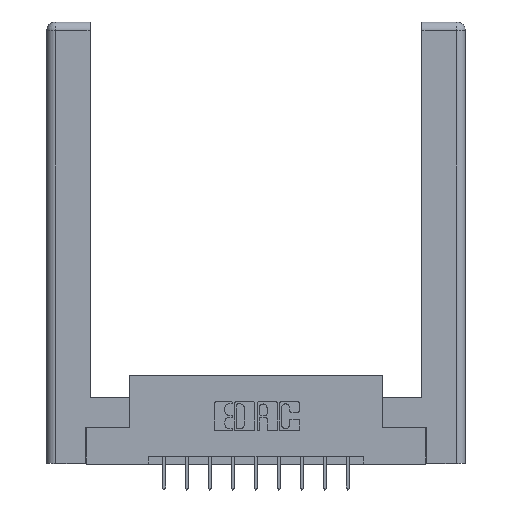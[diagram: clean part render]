
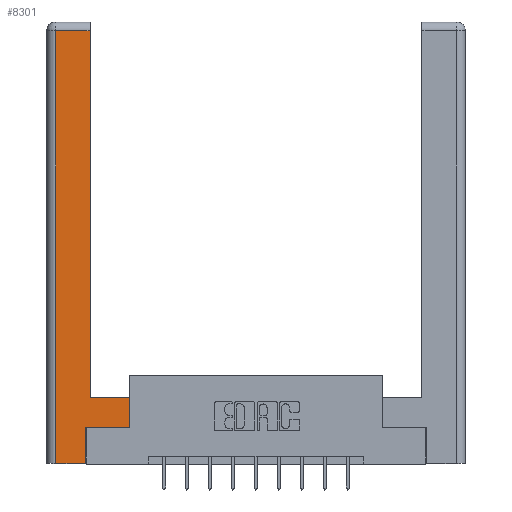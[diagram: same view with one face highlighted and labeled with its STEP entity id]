
A CAD part, top view. The second image highlights one B-rep face of the part: STEP entity #8301.
In plain terms, the highlighted planar face has unit normal (0, 0, 1).
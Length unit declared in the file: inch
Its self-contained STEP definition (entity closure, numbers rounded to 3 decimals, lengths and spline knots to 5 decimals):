
#7 = LINE ( 'NONE', #2999, #8650 ) ;
#474 = CARTESIAN_POINT ( 'NONE',  ( 0.265, 0., 0. ) ) ;
#619 = VERTEX_POINT ( 'NONE', #7147 ) ;
#629 = LINE ( 'NONE', #12788, #7188 ) ;
#759 = CARTESIAN_POINT ( 'NONE',  ( 0.565, 0.45, 0. ) ) ;
#1500 = ORIENTED_EDGE ( 'NONE', *, *, #8595, .T. ) ;
#1801 = VECTOR ( 'NONE', #3894, 39.37008 ) ;
#2249 = LINE ( 'NONE', #9112, #7304 ) ;
#2754 = VERTEX_POINT ( 'NONE', #8415 ) ;
#2829 = LINE ( 'NONE', #7089, #1801 ) ;
#2940 = CARTESIAN_POINT ( 'NONE',  ( 0.565, 0.245, 0. ) ) ;
#2999 = CARTESIAN_POINT ( 'NONE',  ( 0.295, 3., 0. ) ) ;
#3334 = DIRECTION ( 'NONE',  ( -1., 0., 0. ) ) ;
#3894 = DIRECTION ( 'NONE',  ( -1., 0., 0. ) ) ;
#3962 = EDGE_CURVE ( 'NONE', #5078, #12173, #629, .T. ) ;
#4452 = CARTESIAN_POINT ( 'NONE',  ( 0.0615, 2.94, 0. ) ) ;
#4752 = VECTOR ( 'NONE', #6520, 39.37008 ) ;
#4758 = CARTESIAN_POINT ( 'NONE',  ( 0.265, 0.245, 0. ) ) ;
#5025 = LINE ( 'NONE', #12122, #11454 ) ;
#5056 = ORIENTED_EDGE ( 'NONE', *, *, #13034, .T. ) ;
#5078 = VERTEX_POINT ( 'NONE', #2940 ) ;
#5204 = FACE_OUTER_BOUND ( 'NONE', #5707, .T. ) ;
#5498 = VERTEX_POINT ( 'NONE', #11136 ) ;
#5707 = EDGE_LOOP ( 'NONE', ( #13504, #7540, #7844, #9183, #5056, #1500, #11090, #7288 ) ) ;
#5797 = AXIS2_PLACEMENT_3D ( 'NONE', #7119, #11434, #12456 ) ;
#5923 = CARTESIAN_POINT ( 'NONE',  ( 0.295, 0.45, 0. ) ) ;
#6492 = DIRECTION ( 'NONE',  ( 0., 1., 0. ) ) ;
#6520 = DIRECTION ( 'NONE',  ( 1., 0., 0. ) ) ;
#6561 = VERTEX_POINT ( 'NONE', #5923 ) ;
#6956 = EDGE_CURVE ( 'NONE', #2754, #11040, #9475, .T. ) ;
#7089 = CARTESIAN_POINT ( 'NONE',  ( 0.295, 0.45, 0. ) ) ;
#7119 = CARTESIAN_POINT ( 'NONE',  ( 0., 0., 0. ) ) ;
#7147 = CARTESIAN_POINT ( 'NONE',  ( 0.265, 0.245, 0. ) ) ;
#7188 = VECTOR ( 'NONE', #6492, 39.37008 ) ;
#7288 = ORIENTED_EDGE ( 'NONE', *, *, #8622, .T. ) ;
#7304 = VECTOR ( 'NONE', #10137, 39.37008 ) ;
#7540 = ORIENTED_EDGE ( 'NONE', *, *, #7858, .T. ) ;
#7578 = LINE ( 'NONE', #4758, #10715 ) ;
#7844 = ORIENTED_EDGE ( 'NONE', *, *, #11564, .T. ) ;
#7858 = EDGE_CURVE ( 'NONE', #13537, #5498, #10970, .T. ) ;
#8301 = ADVANCED_FACE ( 'NONE', ( #5204 ), #13443, .F. ) ;
#8415 = CARTESIAN_POINT ( 'NONE',  ( 0.0615, 0., 0. ) ) ;
#8595 = EDGE_CURVE ( 'NONE', #619, #5078, #5025, .T. ) ;
#8607 = CARTESIAN_POINT ( 'NONE',  ( 0.265, 0., 0. ) ) ;
#8622 = EDGE_CURVE ( 'NONE', #12173, #6561, #2829, .T. ) ;
#8650 = VECTOR ( 'NONE', #12708, 39.37008 ) ;
#9112 = CARTESIAN_POINT ( 'NONE',  ( 0.0615, 0., 0. ) ) ;
#9183 = ORIENTED_EDGE ( 'NONE', *, *, #6956, .T. ) ;
#9280 = VECTOR ( 'NONE', #3334, 39.37008 ) ;
#9475 = LINE ( 'NONE', #8607, #4752 ) ;
#10137 = DIRECTION ( 'NONE',  ( 0., -1., 0. ) ) ;
#10715 = VECTOR ( 'NONE', #12314, 39.37008 ) ;
#10837 = DIRECTION ( 'NONE',  ( 1., 0., 0. ) ) ;
#10970 = LINE ( 'NONE', #4452, #9280 ) ;
#11040 = VERTEX_POINT ( 'NONE', #474 ) ;
#11090 = ORIENTED_EDGE ( 'NONE', *, *, #3962, .T. ) ;
#11136 = CARTESIAN_POINT ( 'NONE',  ( 0.0615, 2.94, 0. ) ) ;
#11434 = DIRECTION ( 'NONE',  ( 0., 0., -1. ) ) ;
#11454 = VECTOR ( 'NONE', #10837, 39.37008 ) ;
#11564 = EDGE_CURVE ( 'NONE', #5498, #2754, #2249, .T. ) ;
#12122 = CARTESIAN_POINT ( 'NONE',  ( 0.565, 0.245, 0. ) ) ;
#12173 = VERTEX_POINT ( 'NONE', #759 ) ;
#12314 = DIRECTION ( 'NONE',  ( 0., 1., 0. ) ) ;
#12456 = DIRECTION ( 'NONE',  ( -1., 0., 0. ) ) ;
#12708 = DIRECTION ( 'NONE',  ( 0., 1., 0. ) ) ;
#12788 = CARTESIAN_POINT ( 'NONE',  ( 0.565, 0.45, 0. ) ) ;
#12819 = EDGE_CURVE ( 'NONE', #6561, #13537, #7, .T. ) ;
#13034 = EDGE_CURVE ( 'NONE', #11040, #619, #7578, .T. ) ;
#13265 = CARTESIAN_POINT ( 'NONE',  ( 0.295, 2.94, 0. ) ) ;
#13443 = PLANE ( 'NONE',  #5797 ) ;
#13504 = ORIENTED_EDGE ( 'NONE', *, *, #12819, .T. ) ;
#13537 = VERTEX_POINT ( 'NONE', #13265 ) ;
